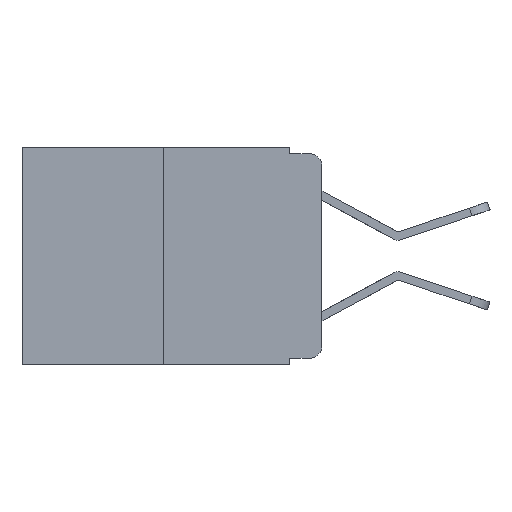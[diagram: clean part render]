
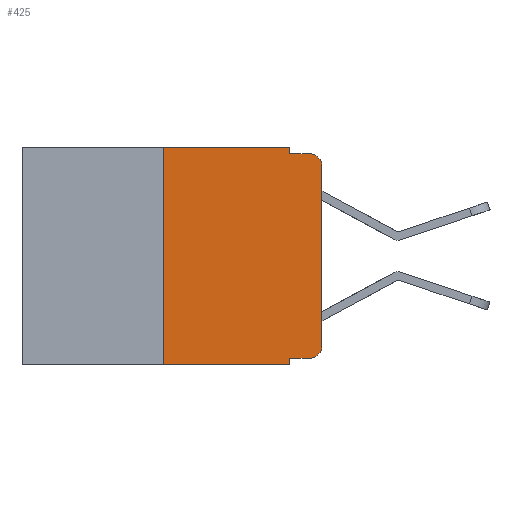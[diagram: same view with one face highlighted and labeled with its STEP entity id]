
A CAD part, left-side view. The second image highlights one B-rep face of the part: STEP entity #425.
In plain terms, the highlighted planar face has unit normal (-1, 0, 0).
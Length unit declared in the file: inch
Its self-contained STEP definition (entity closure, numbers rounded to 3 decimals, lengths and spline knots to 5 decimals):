
#26 = ORIENTED_EDGE ( 'NONE', *, *, #5784, .F. ) ;
#297 = CIRCLE ( 'NONE', #8701, 0.02 ) ;
#343 = CARTESIAN_POINT ( 'NONE',  ( 0., 0.02, -0.03 ) ) ;
#425 = ADVANCED_FACE ( 'NONE', ( #7662 ), #11552, .F. ) ;
#674 = LINE ( 'NONE', #11368, #5475 ) ;
#788 = LINE ( 'NONE', #5697, #3249 ) ;
#915 = CARTESIAN_POINT ( 'NONE',  ( 0., 0.051, 0. ) ) ;
#1300 = ORIENTED_EDGE ( 'NONE', *, *, #4520, .F. ) ;
#1332 = ORIENTED_EDGE ( 'NONE', *, *, #7511, .T. ) ;
#1336 = EDGE_CURVE ( 'NONE', #1595, #2534, #4045, .T. ) ;
#1594 = DIRECTION ( 'NONE',  ( 0., 0., -1. ) ) ;
#1595 = VERTEX_POINT ( 'NONE', #2031 ) ;
#2031 = CARTESIAN_POINT ( 'NONE',  ( 0., 0.25, -0.343 ) ) ;
#2050 = CARTESIAN_POINT ( 'NONE',  ( 0., 0.02, -0.313 ) ) ;
#2154 = VECTOR ( 'NONE', #6795, 39.37008 ) ;
#2396 = EDGE_CURVE ( 'NONE', #3328, #9167, #4782, .T. ) ;
#2534 = VERTEX_POINT ( 'NONE', #7305 ) ;
#2916 = ORIENTED_EDGE ( 'NONE', *, *, #2396, .T. ) ;
#2951 = CARTESIAN_POINT ( 'NONE',  ( 0., 0., 0. ) ) ;
#3172 = EDGE_CURVE ( 'NONE', #9167, #8655, #297, .T. ) ;
#3239 = DIRECTION ( 'NONE',  ( 0., 0., -1. ) ) ;
#3249 = VECTOR ( 'NONE', #6573, 39.37008 ) ;
#3328 = VERTEX_POINT ( 'NONE', #11550 ) ;
#3553 = DIRECTION ( 'NONE',  ( 0., 0., -1. ) ) ;
#3717 = LINE ( 'NONE', #7149, #8183 ) ;
#3981 = ORIENTED_EDGE ( 'NONE', *, *, #3172, .T. ) ;
#3984 = CARTESIAN_POINT ( 'NONE',  ( 0., 0.473, 0. ) ) ;
#4045 = LINE ( 'NONE', #10483, #6282 ) ;
#4285 = ORIENTED_EDGE ( 'NONE', *, *, #10879, .F. ) ;
#4520 = EDGE_CURVE ( 'NONE', #8652, #7895, #674, .T. ) ;
#4782 = LINE ( 'NONE', #2951, #9025 ) ;
#5058 = VERTEX_POINT ( 'NONE', #8602 ) ;
#5060 = CARTESIAN_POINT ( 'NONE',  ( 0., 0.051, -0.01 ) ) ;
#5131 = CIRCLE ( 'NONE', #8453, 0.02 ) ;
#5204 = CARTESIAN_POINT ( 'NONE',  ( 0., 0.02, -0.333 ) ) ;
#5210 = DIRECTION ( 'NONE',  ( 0., -1., 0. ) ) ;
#5289 = CARTESIAN_POINT ( 'NONE',  ( 0., 0.02, -0.01 ) ) ;
#5475 = VECTOR ( 'NONE', #11398, 39.37008 ) ;
#5487 = CARTESIAN_POINT ( 'NONE',  ( 0., 0.051, 0. ) ) ;
#5697 = CARTESIAN_POINT ( 'NONE',  ( 0., 0.25, 0. ) ) ;
#5784 = EDGE_CURVE ( 'NONE', #7895, #8655, #8331, .T. ) ;
#6138 = LINE ( 'NONE', #5487, #8086 ) ;
#6265 = VERTEX_POINT ( 'NONE', #7982 ) ;
#6282 = VECTOR ( 'NONE', #5210, 39.37008 ) ;
#6390 = EDGE_CURVE ( 'NONE', #6265, #2534, #6138, .T. ) ;
#6573 = DIRECTION ( 'NONE',  ( 0., 0., 1. ) ) ;
#6689 = AXIS2_PLACEMENT_3D ( 'NONE', #11326, #11685, #11227 ) ;
#6696 = CARTESIAN_POINT ( 'NONE',  ( 0., 0., -0.03 ) ) ;
#6795 = DIRECTION ( 'NONE',  ( 0., -1., 0. ) ) ;
#7149 = CARTESIAN_POINT ( 'NONE',  ( 0., 0.051, -0.333 ) ) ;
#7305 = CARTESIAN_POINT ( 'NONE',  ( 0., 0.051, -0.343 ) ) ;
#7369 = CARTESIAN_POINT ( 'NONE',  ( 0., 0.051, -0.01 ) ) ;
#7506 = DIRECTION ( 'NONE',  ( -1., 0., 0. ) ) ;
#7511 = EDGE_CURVE ( 'NONE', #6265, #8560, #3717, .T. ) ;
#7662 = FACE_OUTER_BOUND ( 'NONE', #10486, .T. ) ;
#7767 = ORIENTED_EDGE ( 'NONE', *, *, #8055, .F. ) ;
#7895 = VERTEX_POINT ( 'NONE', #7369 ) ;
#7968 = DIRECTION ( 'NONE',  ( 0., -1., 0. ) ) ;
#7982 = CARTESIAN_POINT ( 'NONE',  ( 0., 0.051, -0.333 ) ) ;
#8055 = EDGE_CURVE ( 'NONE', #1595, #5058, #788, .T. ) ;
#8086 = VECTOR ( 'NONE', #3553, 39.37008 ) ;
#8183 = VECTOR ( 'NONE', #7968, 39.37008 ) ;
#8222 = DIRECTION ( 'NONE',  ( 0., 0., 1. ) ) ;
#8331 = LINE ( 'NONE', #5060, #9685 ) ;
#8453 = AXIS2_PLACEMENT_3D ( 'NONE', #2050, #8570, #3239 ) ;
#8559 = EDGE_CURVE ( 'NONE', #8560, #3328, #5131, .T. ) ;
#8560 = VERTEX_POINT ( 'NONE', #5204 ) ;
#8570 = DIRECTION ( 'NONE',  ( -1., 0., 0. ) ) ;
#8602 = CARTESIAN_POINT ( 'NONE',  ( 0., 0.25, 0. ) ) ;
#8652 = VERTEX_POINT ( 'NONE', #915 ) ;
#8655 = VERTEX_POINT ( 'NONE', #5289 ) ;
#8701 = AXIS2_PLACEMENT_3D ( 'NONE', #343, #7506, #1594 ) ;
#8711 = ORIENTED_EDGE ( 'NONE', *, *, #8559, .T. ) ;
#9025 = VECTOR ( 'NONE', #8222, 39.37008 ) ;
#9167 = VERTEX_POINT ( 'NONE', #6696 ) ;
#9232 = DIRECTION ( 'NONE',  ( 0., -1., 0. ) ) ;
#9685 = VECTOR ( 'NONE', #9232, 39.37008 ) ;
#9930 = ORIENTED_EDGE ( 'NONE', *, *, #1336, .T. ) ;
#10483 = CARTESIAN_POINT ( 'NONE',  ( 0., 0.473, -0.343 ) ) ;
#10486 = EDGE_LOOP ( 'NONE', ( #2916, #3981, #26, #1300, #4285, #7767, #9930, #10662, #1332, #8711 ) ) ;
#10662 = ORIENTED_EDGE ( 'NONE', *, *, #6390, .F. ) ;
#10879 = EDGE_CURVE ( 'NONE', #5058, #8652, #11452, .T. ) ;
#11227 = DIRECTION ( 'NONE',  ( 0., 0., -1. ) ) ;
#11326 = CARTESIAN_POINT ( 'NONE',  ( 0., 0.473, 0. ) ) ;
#11368 = CARTESIAN_POINT ( 'NONE',  ( 0., 0.051, 0. ) ) ;
#11398 = DIRECTION ( 'NONE',  ( 0., 0., -1. ) ) ;
#11452 = LINE ( 'NONE', #3984, #2154 ) ;
#11550 = CARTESIAN_POINT ( 'NONE',  ( 0., 0., -0.313 ) ) ;
#11552 = PLANE ( 'NONE',  #6689 ) ;
#11685 = DIRECTION ( 'NONE',  ( 1., 0., 0. ) ) ;
